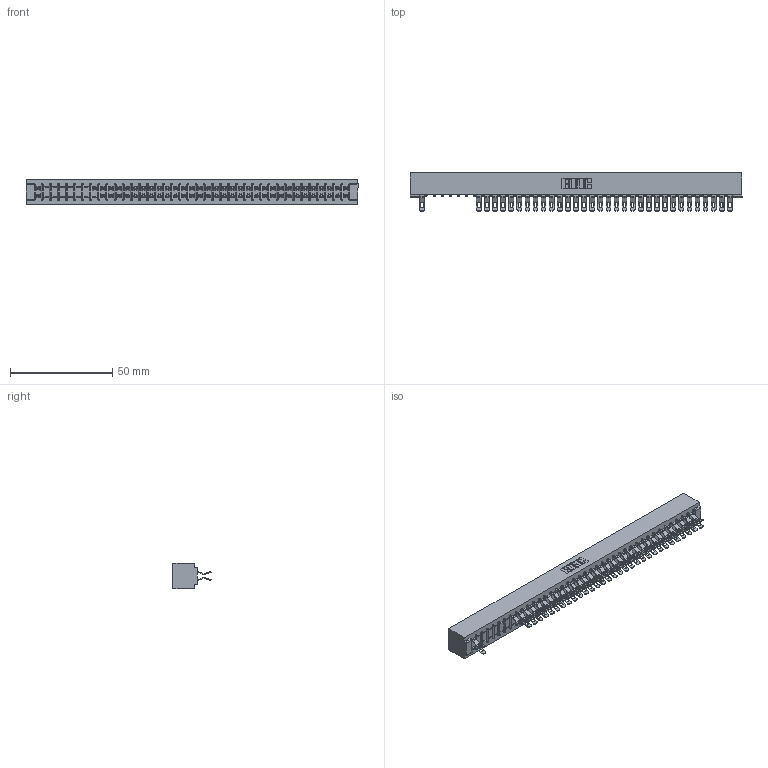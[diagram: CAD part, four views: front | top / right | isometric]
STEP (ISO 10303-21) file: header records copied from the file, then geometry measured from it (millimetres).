
FILE_DESCRIPTION (( 'STEP AP203' ), '1' );
FILE_NAME ('307-078-555-201.STEP', '2018-08-06T17:50:18', ( '' ), ( '' ), 'SwSTEP 2.0', 'SolidWorks 2016', '' );
FILE_SCHEMA (( 'CONFIG_CONTROL_DESIGN' ));
Length unit declared in the file: inch
Products named in the file (3): 307-290-001_555; 307-078-555-201; 307 Part_No Mounting Lugs
Assembly tree (66 placements, depth 2):
  307-078-555-201
    307 Part_No Mounting Lugs
    307-290-001_555  x65
Bounding box: 162.41 x 18.75 x 12.7 mm (x, y, z)
Volume: 17821.8 mm3; surface area: 22029.9 mm2
Topology: 66 solids, 66 shells, 4245 faces, 12480 edges, 8124 vertices
Faces by surface type: plane 2354, cylinder 1811, sphere 80
Entity records: 34895 total; most frequent: CARTESIAN_POINT 5766, ORIENTED_EDGE 5728, DIRECTION 5642, EDGE_CURVE 2864, LINE 2186, VECTOR 2186, VERTEX_POINT 1852, AXIS2_PLACEMENT_3D 1728
